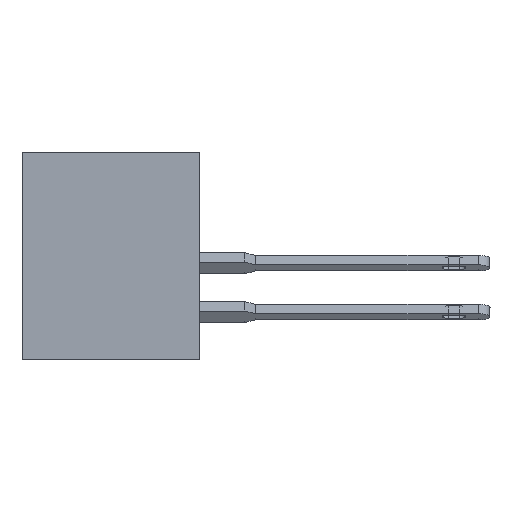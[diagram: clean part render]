
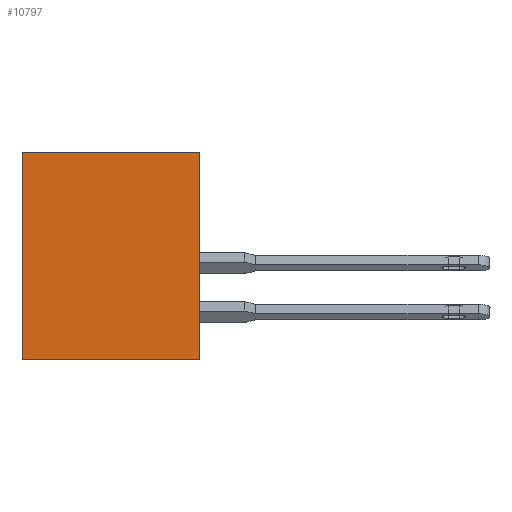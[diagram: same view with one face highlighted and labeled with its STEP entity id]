
A CAD part, left-side view. The second image highlights one B-rep face of the part: STEP entity #10797.
In plain terms, the highlighted planar face has unit normal (-1, 0, 0).
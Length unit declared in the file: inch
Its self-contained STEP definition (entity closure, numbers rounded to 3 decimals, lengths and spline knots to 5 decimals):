
#1161 = DIRECTION ( 'NONE',  ( 1., 0., 0. ) ) ;
#1285 = LINE ( 'NONE', #20668, #3305 ) ;
#1582 = DIRECTION ( 'NONE',  ( 0., 0., 1. ) ) ;
#3305 = VECTOR ( 'NONE', #6079, 39.37008 ) ;
#4380 = DIRECTION ( 'NONE',  ( 0., -1., 0. ) ) ;
#4578 = ORIENTED_EDGE ( 'NONE', *, *, #27429, .F. ) ;
#5252 = DIRECTION ( 'NONE',  ( 0., 0., -1. ) ) ;
#6079 = DIRECTION ( 'NONE',  ( 0., 0., 1. ) ) ;
#7150 = CARTESIAN_POINT ( 'NONE',  ( 0., 0., 0. ) ) ;
#7704 = EDGE_CURVE ( 'NONE', #12008, #9320, #9815, .T. ) ;
#8433 = CARTESIAN_POINT ( 'NONE',  ( 0., 0.453, -0.531 ) ) ;
#8592 = ORIENTED_EDGE ( 'NONE', *, *, #7704, .F. ) ;
#8740 = LINE ( 'NONE', #8433, #13088 ) ;
#9320 = VERTEX_POINT ( 'NONE', #7150 ) ;
#9815 = LINE ( 'NONE', #26057, #25838 ) ;
#10365 = LINE ( 'NONE', #11874, #26407 ) ;
#10797 = ADVANCED_FACE ( 'NONE', ( #22004 ), #13794, .F. ) ;
#11874 = CARTESIAN_POINT ( 'NONE',  ( 0., 0.453, 0. ) ) ;
#12008 = VERTEX_POINT ( 'NONE', #21582 ) ;
#12741 = VERTEX_POINT ( 'NONE', #25575 ) ;
#13088 = VECTOR ( 'NONE', #4380, 39.37008 ) ;
#13794 = PLANE ( 'NONE',  #20424 ) ;
#14109 = ORIENTED_EDGE ( 'NONE', *, *, #27135, .T. ) ;
#15399 = VERTEX_POINT ( 'NONE', #25536 ) ;
#15661 = CARTESIAN_POINT ( 'NONE',  ( 0., 0.453, 0. ) ) ;
#20424 = AXIS2_PLACEMENT_3D ( 'NONE', #15661, #1161, #5252 ) ;
#20668 = CARTESIAN_POINT ( 'NONE',  ( 0., 0., 0. ) ) ;
#21582 = CARTESIAN_POINT ( 'NONE',  ( 0., 0.453, 0. ) ) ;
#21852 = DIRECTION ( 'NONE',  ( 0., -1., 0. ) ) ;
#22004 = FACE_OUTER_BOUND ( 'NONE', #24125, .T. ) ;
#24125 = EDGE_LOOP ( 'NONE', ( #26869, #8592, #4578, #14109 ) ) ;
#24489 = EDGE_CURVE ( 'NONE', #15399, #9320, #1285, .T. ) ;
#25536 = CARTESIAN_POINT ( 'NONE',  ( 0., 0., -0.531 ) ) ;
#25575 = CARTESIAN_POINT ( 'NONE',  ( 0., 0.453, -0.531 ) ) ;
#25838 = VECTOR ( 'NONE', #21852, 39.37008 ) ;
#26057 = CARTESIAN_POINT ( 'NONE',  ( 0., 0.453, 0. ) ) ;
#26407 = VECTOR ( 'NONE', #1582, 39.37008 ) ;
#26869 = ORIENTED_EDGE ( 'NONE', *, *, #24489, .T. ) ;
#27135 = EDGE_CURVE ( 'NONE', #12741, #15399, #8740, .T. ) ;
#27429 = EDGE_CURVE ( 'NONE', #12741, #12008, #10365, .T. ) ;
